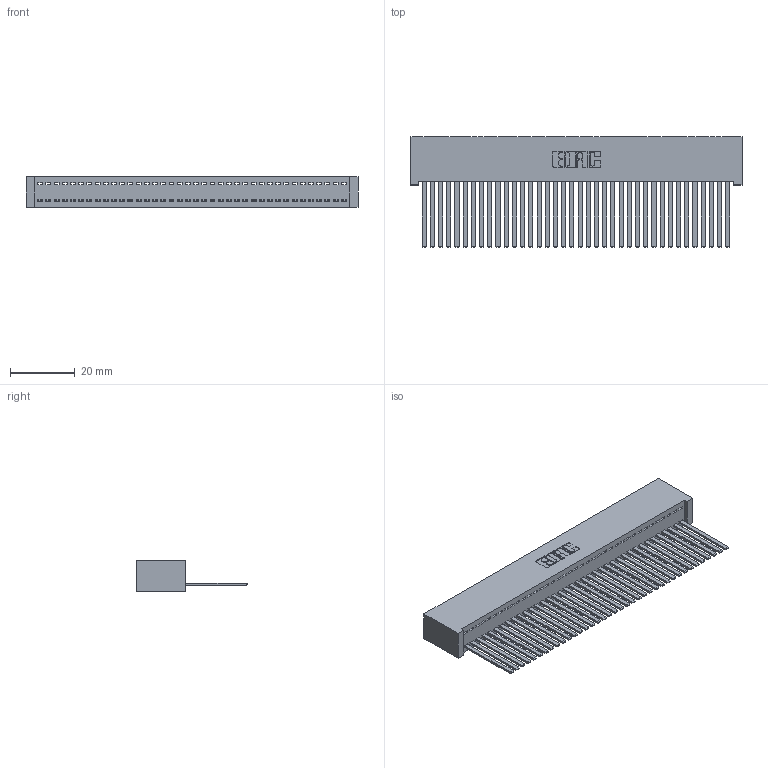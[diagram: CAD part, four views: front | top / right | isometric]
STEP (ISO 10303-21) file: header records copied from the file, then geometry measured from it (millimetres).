
FILE_DESCRIPTION (( 'STEP AP203' ), '1' );
FILE_NAME ('392-038-544-101.STEP', '2018-08-16T05:36:12', ( '' ), ( '' ), 'SwSTEP 2.0', 'SolidWorks 2016', '' );
FILE_SCHEMA (( 'CONFIG_CONTROL_DESIGN' ));
Length unit declared in the file: inch
Products named in the file (3): 342 Part_Lugless; 345-292-001_345-293-144; 392-038-544-101
Assembly tree (39 placements, depth 2):
  392-038-544-101
    342 Part_Lugless
    345-292-001_345-293-144  x38
Bounding box: 102.77 x 34.3 x 9.4 mm (x, y, z)
Volume: 9845.1 mm3; surface area: 15958.2 mm2
Topology: 39 solids, 39 shells, 2078 faces, 6279 edges, 4134 vertices
Faces by surface type: plane 1506, cylinder 572
Entity records: 23155 total; most frequent: CARTESIAN_POINT 4000, ORIENTED_EDGE 3974, DIRECTION 3371, EDGE_CURVE 1987, LINE 1871, VECTOR 1871, VERTEX_POINT 1322, AXIS2_PLACEMENT_3D 750
